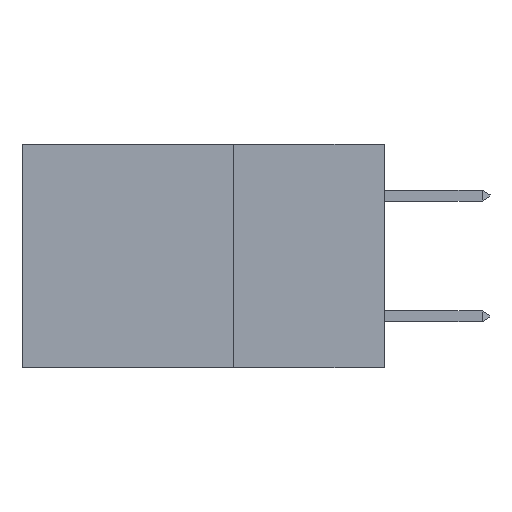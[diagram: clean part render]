
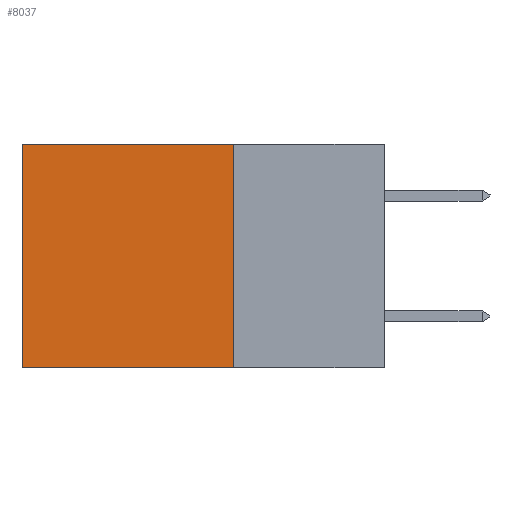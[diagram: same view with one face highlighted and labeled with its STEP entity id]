
A CAD part, left-side view. The second image highlights one B-rep face of the part: STEP entity #8037.
In plain terms, the highlighted planar face has unit normal (-1, 0, 0).
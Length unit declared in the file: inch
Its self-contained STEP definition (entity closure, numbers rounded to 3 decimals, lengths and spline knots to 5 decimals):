
#519 = CARTESIAN_POINT ( 'NONE',  ( 0.2875, 0.25, -0.37 ) ) ;
#1561 = CARTESIAN_POINT ( 'NONE',  ( 0.2875, 0.6, 0. ) ) ;
#1781 = DIRECTION ( 'NONE',  ( 1., 0., 0. ) ) ;
#2567 = LINE ( 'NONE', #519, #28745 ) ;
#4274 = EDGE_CURVE ( 'NONE', #10242, #14175, #21901, .T. ) ;
#5201 = ORIENTED_EDGE ( 'NONE', *, *, #20572, .F. ) ;
#6761 = EDGE_CURVE ( 'NONE', #10242, #12102, #34102, .T. ) ;
#8037 = ADVANCED_FACE ( 'NONE', ( #28070 ), #19132, .F. ) ;
#8337 = AXIS2_PLACEMENT_3D ( 'NONE', #28066, #1781, #28204 ) ;
#8630 = DIRECTION ( 'NONE',  ( 0., 1., 0. ) ) ;
#8705 = ORIENTED_EDGE ( 'NONE', *, *, #6761, .T. ) ;
#9032 = CARTESIAN_POINT ( 'NONE',  ( 0.2875, 0.25, 0. ) ) ;
#9934 = CARTESIAN_POINT ( 'NONE',  ( 0.2875, 0.6, -0.37 ) ) ;
#10242 = VERTEX_POINT ( 'NONE', #10271 ) ;
#10271 = CARTESIAN_POINT ( 'NONE',  ( 0.2875, 0.25, 0. ) ) ;
#11033 = ORIENTED_EDGE ( 'NONE', *, *, #29599, .T. ) ;
#12102 = VERTEX_POINT ( 'NONE', #1561 ) ;
#14175 = VERTEX_POINT ( 'NONE', #32116 ) ;
#19132 = PLANE ( 'NONE',  #8337 ) ;
#20572 = EDGE_CURVE ( 'NONE', #14175, #23628, #2567, .T. ) ;
#20878 = CARTESIAN_POINT ( 'NONE',  ( 0.2875, 0.6, 0. ) ) ;
#21901 = LINE ( 'NONE', #31472, #31020 ) ;
#23628 = VERTEX_POINT ( 'NONE', #9934 ) ;
#26997 = EDGE_LOOP ( 'NONE', ( #11033, #5201, #37440, #8705 ) ) ;
#28066 = CARTESIAN_POINT ( 'NONE',  ( 0.2875, 0.25, 0. ) ) ;
#28070 = FACE_OUTER_BOUND ( 'NONE', #26997, .T. ) ;
#28204 = DIRECTION ( 'NONE',  ( 0., 0., -1. ) ) ;
#28745 = VECTOR ( 'NONE', #35762, 39.37008 ) ;
#28794 = DIRECTION ( 'NONE',  ( 0., 0., -1. ) ) ;
#29599 = EDGE_CURVE ( 'NONE', #12102, #23628, #30832, .T. ) ;
#30832 = LINE ( 'NONE', #20878, #35843 ) ;
#31020 = VECTOR ( 'NONE', #28794, 39.37008 ) ;
#31472 = CARTESIAN_POINT ( 'NONE',  ( 0.2875, 0.25, 0. ) ) ;
#32116 = CARTESIAN_POINT ( 'NONE',  ( 0.2875, 0.25, -0.37 ) ) ;
#32279 = VECTOR ( 'NONE', #8630, 39.37008 ) ;
#34102 = LINE ( 'NONE', #9032, #32279 ) ;
#35630 = DIRECTION ( 'NONE',  ( 0., 0., -1. ) ) ;
#35762 = DIRECTION ( 'NONE',  ( 0., 1., 0. ) ) ;
#35843 = VECTOR ( 'NONE', #35630, 39.37008 ) ;
#37440 = ORIENTED_EDGE ( 'NONE', *, *, #4274, .F. ) ;
